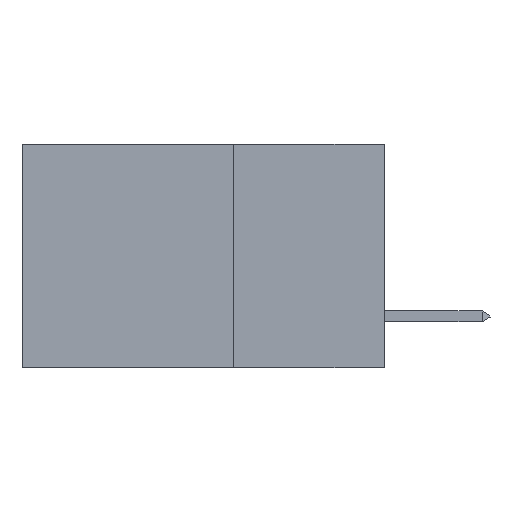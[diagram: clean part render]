
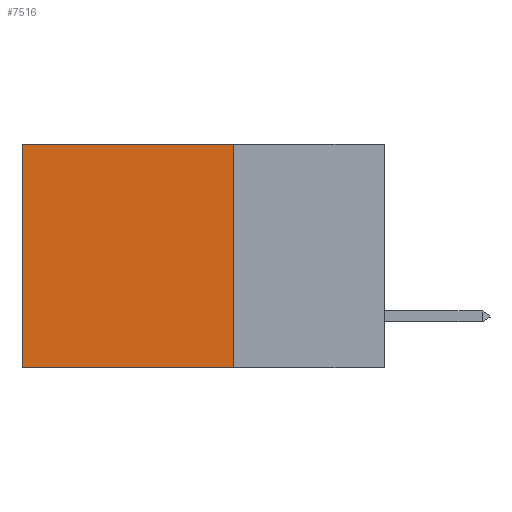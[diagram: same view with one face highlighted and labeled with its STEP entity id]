
A CAD part, left-side view. The second image highlights one B-rep face of the part: STEP entity #7516.
In plain terms, the highlighted planar face has unit normal (-1, 0, 0).
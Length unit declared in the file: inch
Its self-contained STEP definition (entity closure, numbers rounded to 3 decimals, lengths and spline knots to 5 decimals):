
#236 = FACE_OUTER_BOUND ( 'NONE', #40391, .T. ) ;
#424 = VERTEX_POINT ( 'NONE', #6355 ) ;
#629 = DIRECTION ( 'NONE',  ( 1., 0., 0. ) ) ;
#2092 = ORIENTED_EDGE ( 'NONE', *, *, #17880, .T. ) ;
#2221 = CARTESIAN_POINT ( 'NONE',  ( 0.2875, 0.6, -0.37 ) ) ;
#3285 = CARTESIAN_POINT ( 'NONE',  ( 0.2875, 0.25, 0. ) ) ;
#6355 = CARTESIAN_POINT ( 'NONE',  ( 0.2875, 0.6, 0. ) ) ;
#7516 = ADVANCED_FACE ( 'NONE', ( #236 ), #16176, .F. ) ;
#8013 = LINE ( 'NONE', #33983, #35394 ) ;
#8099 = CARTESIAN_POINT ( 'NONE',  ( 0.2875, 0.25, 0. ) ) ;
#8362 = CARTESIAN_POINT ( 'NONE',  ( 0.2875, 0.25, 0. ) ) ;
#8708 = EDGE_CURVE ( 'NONE', #28199, #19581, #34316, .T. ) ;
#9936 = DIRECTION ( 'NONE',  ( 0., 0., -1. ) ) ;
#12859 = VECTOR ( 'NONE', #35784, 39.37008 ) ;
#13212 = VECTOR ( 'NONE', #21061, 39.37008 ) ;
#14708 = ORIENTED_EDGE ( 'NONE', *, *, #8708, .F. ) ;
#14788 = DIRECTION ( 'NONE',  ( 0., 1., 0. ) ) ;
#16083 = EDGE_CURVE ( 'NONE', #28199, #424, #8013, .T. ) ;
#16176 = PLANE ( 'NONE',  #29718 ) ;
#16338 = CARTESIAN_POINT ( 'NONE',  ( 0.2875, 0.25, -0.37 ) ) ;
#16850 = DIRECTION ( 'NONE',  ( 0., 0., -1. ) ) ;
#17880 = EDGE_CURVE ( 'NONE', #424, #34252, #27968, .T. ) ;
#18939 = LINE ( 'NONE', #16338, #12859 ) ;
#19581 = VERTEX_POINT ( 'NONE', #23760 ) ;
#21061 = DIRECTION ( 'NONE',  ( 0., 0., -1. ) ) ;
#23760 = CARTESIAN_POINT ( 'NONE',  ( 0.2875, 0.25, -0.37 ) ) ;
#25047 = EDGE_CURVE ( 'NONE', #19581, #34252, #18939, .T. ) ;
#27968 = LINE ( 'NONE', #38710, #39969 ) ;
#28199 = VERTEX_POINT ( 'NONE', #8099 ) ;
#29718 = AXIS2_PLACEMENT_3D ( 'NONE', #3285, #629, #16850 ) ;
#30286 = ORIENTED_EDGE ( 'NONE', *, *, #16083, .T. ) ;
#32257 = ORIENTED_EDGE ( 'NONE', *, *, #25047, .F. ) ;
#33983 = CARTESIAN_POINT ( 'NONE',  ( 0.2875, 0.25, 0. ) ) ;
#34252 = VERTEX_POINT ( 'NONE', #2221 ) ;
#34316 = LINE ( 'NONE', #8362, #13212 ) ;
#35394 = VECTOR ( 'NONE', #14788, 39.37008 ) ;
#35784 = DIRECTION ( 'NONE',  ( 0., 1., 0. ) ) ;
#38710 = CARTESIAN_POINT ( 'NONE',  ( 0.2875, 0.6, 0. ) ) ;
#39969 = VECTOR ( 'NONE', #9936, 39.37008 ) ;
#40391 = EDGE_LOOP ( 'NONE', ( #2092, #32257, #14708, #30286 ) ) ;
